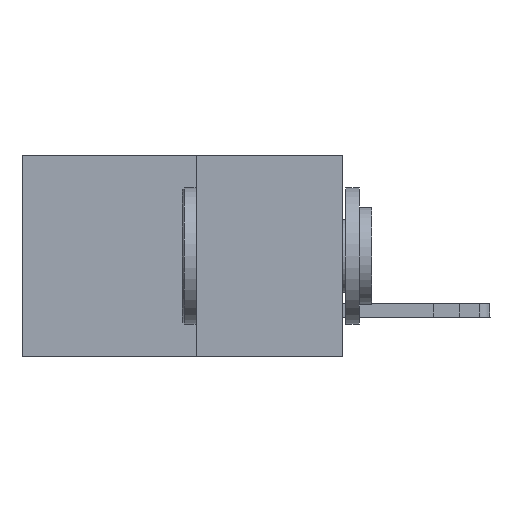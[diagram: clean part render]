
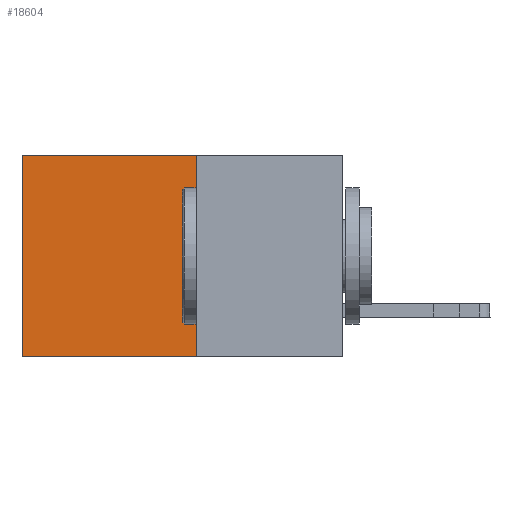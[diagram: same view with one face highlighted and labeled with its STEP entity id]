
A CAD part, left-side view. The second image highlights one B-rep face of the part: STEP entity #18604.
In plain terms, the highlighted planar face has unit normal (-1, 0, 0).
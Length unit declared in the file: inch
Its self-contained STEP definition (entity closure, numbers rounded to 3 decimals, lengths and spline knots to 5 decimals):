
#451 = DIRECTION ( 'NONE',  ( 0., 1., 0. ) ) ;
#571 = ORIENTED_EDGE ( 'NONE', *, *, #15827, .T. ) ;
#1667 = ORIENTED_EDGE ( 'NONE', *, *, #15910, .F. ) ;
#2234 = VECTOR ( 'NONE', #18584, 39.37008 ) ;
#3817 = VECTOR ( 'NONE', #15969, 39.37008 ) ;
#4218 = CARTESIAN_POINT ( 'NONE',  ( 0.277, 0.59, -0.37 ) ) ;
#4344 = EDGE_LOOP ( 'NONE', ( #571, #1667, #6387, #18223 ) ) ;
#4431 = CARTESIAN_POINT ( 'NONE',  ( 0.277, 0.27, -0.37 ) ) ;
#5166 = CARTESIAN_POINT ( 'NONE',  ( 0.277, 0.27, -0.37 ) ) ;
#5428 = VERTEX_POINT ( 'NONE', #17963 ) ;
#5497 = CARTESIAN_POINT ( 'NONE',  ( 0.277, 0.27, 0. ) ) ;
#6087 = VERTEX_POINT ( 'NONE', #4218 ) ;
#6387 = ORIENTED_EDGE ( 'NONE', *, *, #8933, .F. ) ;
#7628 = CARTESIAN_POINT ( 'NONE',  ( 0.277, 0.27, -0.37 ) ) ;
#7812 = EDGE_CURVE ( 'NONE', #8719, #15268, #12821, .T. ) ;
#8642 = LINE ( 'NONE', #4431, #16096 ) ;
#8719 = VERTEX_POINT ( 'NONE', #5497 ) ;
#8933 = EDGE_CURVE ( 'NONE', #8719, #5428, #8642, .T. ) ;
#10591 = LINE ( 'NONE', #7628, #16336 ) ;
#11122 = CARTESIAN_POINT ( 'NONE',  ( 0.277, 0.59, 0. ) ) ;
#12821 = LINE ( 'NONE', #17329, #2234 ) ;
#14490 = DIRECTION ( 'NONE',  ( 0., 0., -1. ) ) ;
#14622 = CARTESIAN_POINT ( 'NONE',  ( 0.277, 0.59, -0.37 ) ) ;
#15268 = VERTEX_POINT ( 'NONE', #11122 ) ;
#15762 = FACE_OUTER_BOUND ( 'NONE', #4344, .T. ) ;
#15827 = EDGE_CURVE ( 'NONE', #15268, #6087, #16249, .T. ) ;
#15910 = EDGE_CURVE ( 'NONE', #5428, #6087, #10591, .T. ) ;
#15969 = DIRECTION ( 'NONE',  ( 0., 0., -1. ) ) ;
#16096 = VECTOR ( 'NONE', #14490, 39.37008 ) ;
#16249 = LINE ( 'NONE', #14622, #3817 ) ;
#16336 = VECTOR ( 'NONE', #451, 39.37008 ) ;
#17122 = AXIS2_PLACEMENT_3D ( 'NONE', #5166, #18288, #18726 ) ;
#17329 = CARTESIAN_POINT ( 'NONE',  ( 0.277, 0.27, 0. ) ) ;
#17963 = CARTESIAN_POINT ( 'NONE',  ( 0.277, 0.27, -0.37 ) ) ;
#18091 = PLANE ( 'NONE',  #17122 ) ;
#18223 = ORIENTED_EDGE ( 'NONE', *, *, #7812, .T. ) ;
#18288 = DIRECTION ( 'NONE',  ( 1., 0., 0. ) ) ;
#18584 = DIRECTION ( 'NONE',  ( 0., 1., 0. ) ) ;
#18604 = ADVANCED_FACE ( 'NONE', ( #15762 ), #18091, .F. ) ;
#18726 = DIRECTION ( 'NONE',  ( 0., 0., -1. ) ) ;
